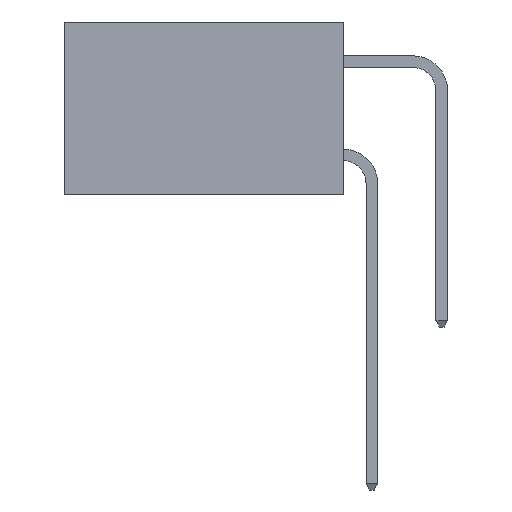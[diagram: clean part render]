
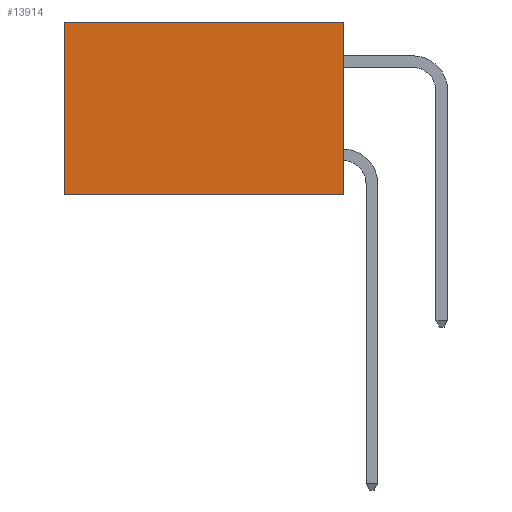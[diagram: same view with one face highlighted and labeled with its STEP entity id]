
A CAD part, left-side view. The second image highlights one B-rep face of the part: STEP entity #13914.
In plain terms, the highlighted planar face has unit normal (-1, 0, 0).
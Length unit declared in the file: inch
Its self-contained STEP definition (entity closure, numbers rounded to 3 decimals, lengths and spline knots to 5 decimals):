
#36 = DIRECTION ( 'NONE',  ( 0., 0., -1. ) ) ;
#59 = LINE ( 'NONE', #267, #7554 ) ;
#267 = CARTESIAN_POINT ( 'NONE',  ( 0.2615, 0.6, -0.37 ) ) ;
#379 = CARTESIAN_POINT ( 'NONE',  ( 0.2615, 0., 0. ) ) ;
#572 = VERTEX_POINT ( 'NONE', #379 ) ;
#1931 = DIRECTION ( 'NONE',  ( 0., 0., -1. ) ) ;
#2316 = FACE_OUTER_BOUND ( 'NONE', #14362, .T. ) ;
#3285 = CARTESIAN_POINT ( 'NONE',  ( 0.2615, 0.6, -0.37 ) ) ;
#3490 = CARTESIAN_POINT ( 'NONE',  ( 0.2615, 0., -0.37 ) ) ;
#3549 = VECTOR ( 'NONE', #1931, 39.37008 ) ;
#4383 = LINE ( 'NONE', #14747, #11539 ) ;
#4609 = CARTESIAN_POINT ( 'NONE',  ( 0.2615, 0.6, 0. ) ) ;
#4663 = EDGE_CURVE ( 'NONE', #8440, #10018, #5305, .T. ) ;
#5305 = LINE ( 'NONE', #16511, #12862 ) ;
#6343 = DIRECTION ( 'NONE',  ( 0., 1., 0. ) ) ;
#6683 = EDGE_CURVE ( 'NONE', #9257, #10018, #59, .T. ) ;
#6925 = CARTESIAN_POINT ( 'NONE',  ( 0.2615, 0., -0.37 ) ) ;
#7554 = VECTOR ( 'NONE', #36, 39.37008 ) ;
#7714 = ORIENTED_EDGE ( 'NONE', *, *, #18466, .F. ) ;
#8440 = VERTEX_POINT ( 'NONE', #6925 ) ;
#9257 = VERTEX_POINT ( 'NONE', #4609 ) ;
#9323 = ORIENTED_EDGE ( 'NONE', *, *, #4663, .F. ) ;
#9543 = DIRECTION ( 'NONE',  ( 0., 0., -1. ) ) ;
#9874 = AXIS2_PLACEMENT_3D ( 'NONE', #10852, #18076, #9543 ) ;
#10018 = VERTEX_POINT ( 'NONE', #3285 ) ;
#10852 = CARTESIAN_POINT ( 'NONE',  ( 0.2615, 0., -0.37 ) ) ;
#11539 = VECTOR ( 'NONE', #6343, 39.37008 ) ;
#12862 = VECTOR ( 'NONE', #16510, 39.37008 ) ;
#13914 = ADVANCED_FACE ( 'NONE', ( #2316 ), #16618, .F. ) ;
#14362 = EDGE_LOOP ( 'NONE', ( #17608, #9323, #7714, #16094 ) ) ;
#14476 = EDGE_CURVE ( 'NONE', #572, #9257, #4383, .T. ) ;
#14747 = CARTESIAN_POINT ( 'NONE',  ( 0.2615, 0., 0. ) ) ;
#15001 = LINE ( 'NONE', #3490, #3549 ) ;
#16094 = ORIENTED_EDGE ( 'NONE', *, *, #14476, .T. ) ;
#16510 = DIRECTION ( 'NONE',  ( 0., 1., 0. ) ) ;
#16511 = CARTESIAN_POINT ( 'NONE',  ( 0.2615, 0., -0.37 ) ) ;
#16618 = PLANE ( 'NONE',  #9874 ) ;
#17608 = ORIENTED_EDGE ( 'NONE', *, *, #6683, .T. ) ;
#18076 = DIRECTION ( 'NONE',  ( 1., 0., 0. ) ) ;
#18466 = EDGE_CURVE ( 'NONE', #572, #8440, #15001, .T. ) ;
